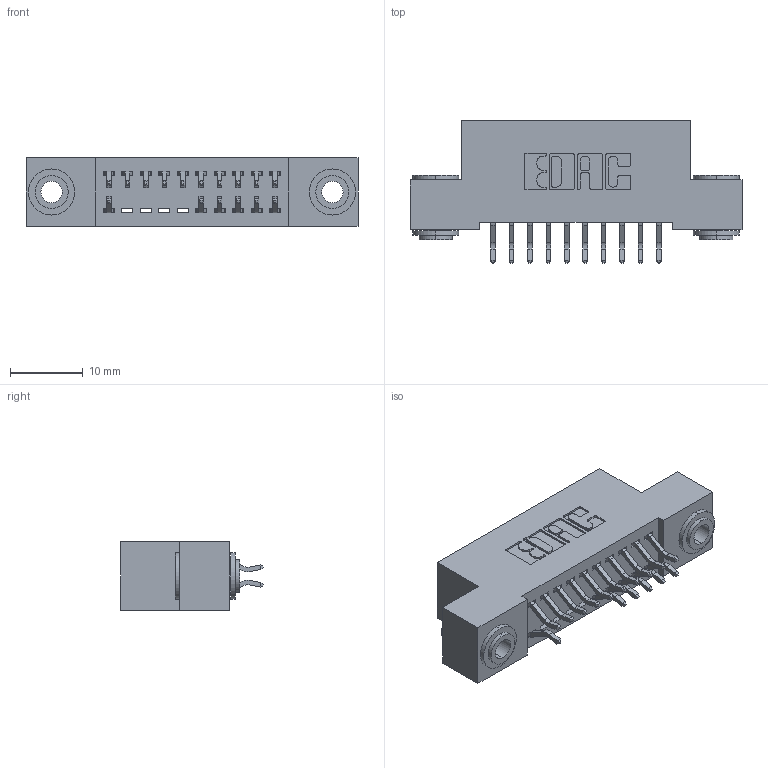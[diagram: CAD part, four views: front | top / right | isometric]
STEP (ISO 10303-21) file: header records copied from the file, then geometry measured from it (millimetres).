
FILE_DESCRIPTION (( 'STEP AP203' ), '1' );
FILE_NAME ('392-020-556-203.STEP', '2018-08-15T07:06:13', ( '' ), ( '' ), 'SwSTEP 2.0', 'SolidWorks 2016', '' );
FILE_SCHEMA (( 'CONFIG_CONTROL_DESIGN' ));
Length unit declared in the file: inch
Products named in the file (4): 342 Part_.156 TH; 345-292-001_556 Tail; 342-250-002_345-250-002-102; 392-020-556-203
Assembly tree (19 placements, depth 2):
  392-020-556-203
    342 Part_.156 TH
    345-292-001_556 Tail  x16
    342-250-002_345-250-002-102  x2
Bounding box: 45.72 x 19.58 x 9.4 mm (x, y, z)
Volume: 3942.9 mm3; surface area: 5629.1 mm2
Topology: 19 solids, 19 shells, 1100 faces, 3227 edges, 2126 vertices
Faces by surface type: plane 740, cylinder 352, cone 8
Entity records: 11182 total; most frequent: CARTESIAN_POINT 1897, ORIENTED_EDGE 1818, DIRECTION 1695, EDGE_CURVE 909, VECTOR 749, LINE 749, VERTEX_POINT 602, AXIS2_PLACEMENT_3D 473
